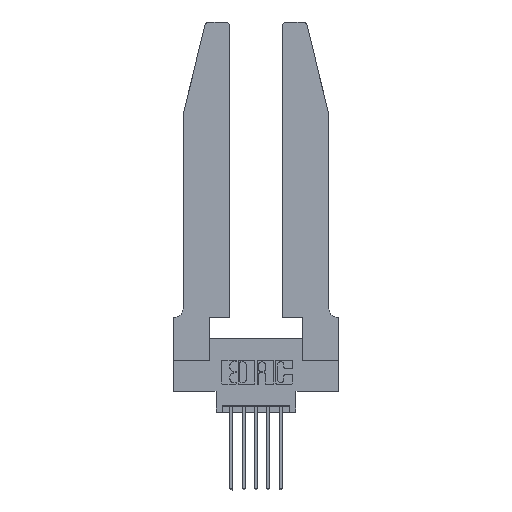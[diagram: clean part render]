
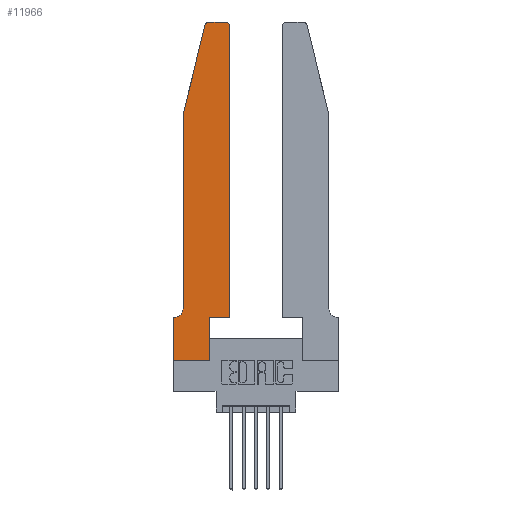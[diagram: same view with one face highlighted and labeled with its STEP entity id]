
A CAD part, top view. The second image highlights one B-rep face of the part: STEP entity #11966.
In plain terms, the highlighted planar face has unit normal (0, 0, 1).
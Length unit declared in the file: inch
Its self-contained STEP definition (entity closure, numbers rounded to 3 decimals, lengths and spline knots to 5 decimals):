
#23 = DIRECTION ( 'NONE',  ( -1., 0., 0. ) ) ;
#278 = EDGE_CURVE ( 'NONE', #502, #5571, #2905, .T. ) ;
#354 = EDGE_CURVE ( 'NONE', #4097, #502, #7201, .T. ) ;
#420 = VECTOR ( 'NONE', #23, 39.37008 ) ;
#502 = VERTEX_POINT ( 'NONE', #5630 ) ;
#643 = FACE_OUTER_BOUND ( 'NONE', #7530, .T. ) ;
#790 = VERTEX_POINT ( 'NONE', #4045 ) ;
#794 = EDGE_CURVE ( 'NONE', #10773, #4509, #7692, .T. ) ;
#987 = VERTEX_POINT ( 'NONE', #12961 ) ;
#1064 = AXIS2_PLACEMENT_3D ( 'NONE', #6084, #13612, #7165 ) ;
#1091 = ORIENTED_EDGE ( 'NONE', *, *, #8365, .T. ) ;
#1205 = VERTEX_POINT ( 'NONE', #1905 ) ;
#1596 = VECTOR ( 'NONE', #13296, 39.37008 ) ;
#1664 = ORIENTED_EDGE ( 'NONE', *, *, #11371, .T. ) ;
#1746 = DIRECTION ( 'NONE',  ( -0.239, -0.971, 0. ) ) ;
#1751 = CARTESIAN_POINT ( 'NONE',  ( 0.4205, 2.72, 0.37 ) ) ;
#1896 = CARTESIAN_POINT ( 'NONE',  ( 0.0755, 2., 0.37 ) ) ;
#1905 = CARTESIAN_POINT ( 'NONE',  ( 0.284, 2.75, 0.37 ) ) ;
#2193 = CIRCLE ( 'NONE', #13791, 0.03 ) ;
#2323 = EDGE_CURVE ( 'NONE', #4254, #6396, #12425, .T. ) ;
#2493 = VECTOR ( 'NONE', #13289, 39.37008 ) ;
#2831 = ORIENTED_EDGE ( 'NONE', *, *, #354, .T. ) ;
#2843 = DIRECTION ( 'NONE',  ( 0., 0., 1. ) ) ;
#2905 = LINE ( 'NONE', #3219, #420 ) ;
#3219 = CARTESIAN_POINT ( 'NONE',  ( 0.0755, 0.35, 0.37 ) ) ;
#3544 = CARTESIAN_POINT ( 'NONE',  ( 0.4505, 0.35, 0.37 ) ) ;
#3768 = EDGE_CURVE ( 'NONE', #6796, #1205, #7648, .T. ) ;
#4045 = CARTESIAN_POINT ( 'NONE',  ( 0.4505, 2.72, 0.37 ) ) ;
#4097 = VERTEX_POINT ( 'NONE', #13730 ) ;
#4135 = CARTESIAN_POINT ( 'NONE',  ( 0.0755, 2., 0.37 ) ) ;
#4254 = VERTEX_POINT ( 'NONE', #5257 ) ;
#4309 = DIRECTION ( 'NONE',  ( -1., 0., 0. ) ) ;
#4329 = LINE ( 'NONE', #12089, #2493 ) ;
#4509 = VERTEX_POINT ( 'NONE', #1896 ) ;
#4527 = EDGE_CURVE ( 'NONE', #790, #6796, #2193, .T. ) ;
#4595 = VERTEX_POINT ( 'NONE', #11568 ) ;
#5056 = LINE ( 'NONE', #7625, #7874 ) ;
#5186 = VECTOR ( 'NONE', #7350, 39.37008 ) ;
#5257 = CARTESIAN_POINT ( 'NONE',  ( 0.2865, 0.35, 0.37 ) ) ;
#5267 = CARTESIAN_POINT ( 'NONE',  ( 0.0055, 0.42, 0.37 ) ) ;
#5571 = VERTEX_POINT ( 'NONE', #9480 ) ;
#5630 = CARTESIAN_POINT ( 'NONE',  ( 0.0055, 0.35, 0.37 ) ) ;
#5789 = CARTESIAN_POINT ( 'NONE',  ( 0.4505, 0.35, 0.37 ) ) ;
#6084 = CARTESIAN_POINT ( 'NONE',  ( 0.284, 2.72, 0.37 ) ) ;
#6307 = DIRECTION ( 'NONE',  ( 0., 0., -1. ) ) ;
#6396 = VERTEX_POINT ( 'NONE', #6596 ) ;
#6435 = EDGE_CURVE ( 'NONE', #5571, #987, #9607, .T. ) ;
#6596 = CARTESIAN_POINT ( 'NONE',  ( 0.4505, 0.35, 0.37 ) ) ;
#6639 = AXIS2_PLACEMENT_3D ( 'NONE', #12504, #7080, #11328 ) ;
#6796 = VERTEX_POINT ( 'NONE', #10258 ) ;
#7080 = DIRECTION ( 'NONE',  ( 0., 0., 1. ) ) ;
#7122 = ORIENTED_EDGE ( 'NONE', *, *, #6435, .T. ) ;
#7165 = DIRECTION ( 'NONE',  ( 1., 0., 0. ) ) ;
#7201 = CIRCLE ( 'NONE', #11604, 0.07 ) ;
#7350 = DIRECTION ( 'NONE',  ( 0., -1., 0. ) ) ;
#7386 = LINE ( 'NONE', #4135, #5186 ) ;
#7530 = EDGE_LOOP ( 'NONE', ( #12570, #11705, #7611, #9116, #2831, #12407, #7122, #1664, #1091, #8588, #7689, #9241 ) ) ;
#7611 = ORIENTED_EDGE ( 'NONE', *, *, #794, .T. ) ;
#7625 = CARTESIAN_POINT ( 'NONE',  ( 0.2865, 0.35, 0.37 ) ) ;
#7628 = EDGE_CURVE ( 'NONE', #6396, #790, #9406, .T. ) ;
#7648 = LINE ( 'NONE', #7716, #8666 ) ;
#7689 = ORIENTED_EDGE ( 'NONE', *, *, #7628, .T. ) ;
#7692 = LINE ( 'NONE', #11330, #8042 ) ;
#7716 = CARTESIAN_POINT ( 'NONE',  ( 0.2605, 2.75, 0.37 ) ) ;
#7874 = VECTOR ( 'NONE', #11795, 39.37008 ) ;
#8042 = VECTOR ( 'NONE', #1746, 39.37008 ) ;
#8129 = CARTESIAN_POINT ( 'NONE',  ( 0.25487, 2.72718, 0.37 ) ) ;
#8203 = EDGE_CURVE ( 'NONE', #4509, #4097, #7386, .T. ) ;
#8365 = EDGE_CURVE ( 'NONE', #4595, #4254, #5056, .T. ) ;
#8588 = ORIENTED_EDGE ( 'NONE', *, *, #2323, .T. ) ;
#8666 = VECTOR ( 'NONE', #13141, 39.37008 ) ;
#8932 = VECTOR ( 'NONE', #9020, 39.37008 ) ;
#9020 = DIRECTION ( 'NONE',  ( 0., -1., 0. ) ) ;
#9116 = ORIENTED_EDGE ( 'NONE', *, *, #8203, .T. ) ;
#9241 = ORIENTED_EDGE ( 'NONE', *, *, #4527, .T. ) ;
#9406 = LINE ( 'NONE', #5789, #1596 ) ;
#9480 = CARTESIAN_POINT ( 'NONE',  ( 0., 0.35, 0.37 ) ) ;
#9607 = LINE ( 'NONE', #13275, #8932 ) ;
#9887 = EDGE_CURVE ( 'NONE', #1205, #10773, #11224, .T. ) ;
#10258 = CARTESIAN_POINT ( 'NONE',  ( 0.4205, 2.75, 0.37 ) ) ;
#10773 = VERTEX_POINT ( 'NONE', #8129 ) ;
#11033 = DIRECTION ( 'NONE',  ( 1., 0., 0. ) ) ;
#11224 = CIRCLE ( 'NONE', #1064, 0.03 ) ;
#11328 = DIRECTION ( 'NONE',  ( 1., 0., 0. ) ) ;
#11330 = CARTESIAN_POINT ( 'NONE',  ( 0.0755, 2., 0.37 ) ) ;
#11371 = EDGE_CURVE ( 'NONE', #987, #4595, #4329, .T. ) ;
#11383 = DIRECTION ( 'NONE',  ( 1., 0., 0. ) ) ;
#11568 = CARTESIAN_POINT ( 'NONE',  ( 0.2865, 0., 0.37 ) ) ;
#11604 = AXIS2_PLACEMENT_3D ( 'NONE', #5267, #6307, #4309 ) ;
#11705 = ORIENTED_EDGE ( 'NONE', *, *, #9887, .T. ) ;
#11752 = VECTOR ( 'NONE', #11033, 39.37008 ) ;
#11795 = DIRECTION ( 'NONE',  ( 0., 1., 0. ) ) ;
#11966 = ADVANCED_FACE ( 'NONE', ( #643 ), #13521, .T. ) ;
#12089 = CARTESIAN_POINT ( 'NONE',  ( 0., 0., 0.37 ) ) ;
#12407 = ORIENTED_EDGE ( 'NONE', *, *, #278, .T. ) ;
#12425 = LINE ( 'NONE', #3544, #11752 ) ;
#12504 = CARTESIAN_POINT ( 'NONE',  ( 0., 0.35, 0.37 ) ) ;
#12570 = ORIENTED_EDGE ( 'NONE', *, *, #3768, .T. ) ;
#12961 = CARTESIAN_POINT ( 'NONE',  ( 0., 0., 0.37 ) ) ;
#13141 = DIRECTION ( 'NONE',  ( -1., 0., 0. ) ) ;
#13275 = CARTESIAN_POINT ( 'NONE',  ( 0., 0., 0.37 ) ) ;
#13289 = DIRECTION ( 'NONE',  ( 1., 0., 0. ) ) ;
#13296 = DIRECTION ( 'NONE',  ( 0., 1., 0. ) ) ;
#13521 = PLANE ( 'NONE',  #6639 ) ;
#13612 = DIRECTION ( 'NONE',  ( 0., 0., 1. ) ) ;
#13730 = CARTESIAN_POINT ( 'NONE',  ( 0.0755, 0.42, 0.37 ) ) ;
#13791 = AXIS2_PLACEMENT_3D ( 'NONE', #1751, #2843, #11383 ) ;
